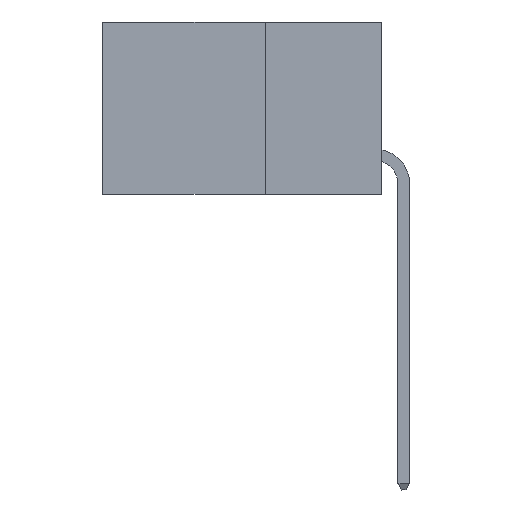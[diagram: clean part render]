
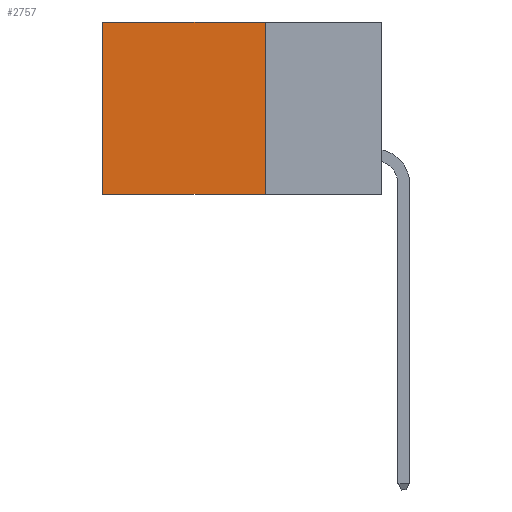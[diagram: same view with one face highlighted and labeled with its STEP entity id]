
A CAD part, left-side view. The second image highlights one B-rep face of the part: STEP entity #2757.
In plain terms, the highlighted planar face has unit normal (-1, 0, 0).
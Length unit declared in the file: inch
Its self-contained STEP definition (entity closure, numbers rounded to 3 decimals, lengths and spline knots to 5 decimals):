
#496 = VECTOR ( 'NONE', #20846, 39.37008 ) ;
#2757 = ADVANCED_FACE ( 'NONE', ( #13807 ), #6725, .F. ) ;
#4314 = DIRECTION ( 'NONE',  ( 0., 1., 0. ) ) ;
#4666 = DIRECTION ( 'NONE',  ( 1., 0., 0. ) ) ;
#4694 = CARTESIAN_POINT ( 'NONE',  ( 0.2875, 0.6, -0.37 ) ) ;
#5157 = CARTESIAN_POINT ( 'NONE',  ( 0.2875, 0.25, -0.37 ) ) ;
#5217 = CARTESIAN_POINT ( 'NONE',  ( 0.2875, 0.6, 0. ) ) ;
#5674 = CARTESIAN_POINT ( 'NONE',  ( 0.2875, 0.25, 0. ) ) ;
#5917 = CARTESIAN_POINT ( 'NONE',  ( 0.2875, 0.25, 0. ) ) ;
#5954 = LINE ( 'NONE', #18958, #496 ) ;
#6725 = PLANE ( 'NONE',  #16886 ) ;
#6920 = LINE ( 'NONE', #5157, #16389 ) ;
#7125 = DIRECTION ( 'NONE',  ( 0., 1., 0. ) ) ;
#7390 = ORIENTED_EDGE ( 'NONE', *, *, #8029, .T. ) ;
#8029 = EDGE_CURVE ( 'NONE', #12331, #22048, #12117, .T. ) ;
#8047 = ORIENTED_EDGE ( 'NONE', *, *, #9166, .T. ) ;
#8820 = DIRECTION ( 'NONE',  ( 0., 0., -1. ) ) ;
#9166 = EDGE_CURVE ( 'NONE', #22048, #13094, #17366, .T. ) ;
#9544 = CARTESIAN_POINT ( 'NONE',  ( 0.2875, 0.6, 0. ) ) ;
#10105 = EDGE_LOOP ( 'NONE', ( #8047, #24276, #16739, #7390 ) ) ;
#11442 = DIRECTION ( 'NONE',  ( 0., 0., -1. ) ) ;
#11542 = VECTOR ( 'NONE', #4314, 39.37008 ) ;
#12117 = LINE ( 'NONE', #17631, #11542 ) ;
#12331 = VERTEX_POINT ( 'NONE', #5917 ) ;
#13094 = VERTEX_POINT ( 'NONE', #4694 ) ;
#13807 = FACE_OUTER_BOUND ( 'NONE', #10105, .T. ) ;
#14584 = EDGE_CURVE ( 'NONE', #19095, #13094, #6920, .T. ) ;
#15245 = EDGE_CURVE ( 'NONE', #12331, #19095, #5954, .T. ) ;
#16175 = VECTOR ( 'NONE', #11442, 39.37008 ) ;
#16389 = VECTOR ( 'NONE', #7125, 39.37008 ) ;
#16739 = ORIENTED_EDGE ( 'NONE', *, *, #15245, .F. ) ;
#16886 = AXIS2_PLACEMENT_3D ( 'NONE', #5674, #4666, #8820 ) ;
#17366 = LINE ( 'NONE', #9544, #16175 ) ;
#17631 = CARTESIAN_POINT ( 'NONE',  ( 0.2875, 0.25, 0. ) ) ;
#18958 = CARTESIAN_POINT ( 'NONE',  ( 0.2875, 0.25, 0. ) ) ;
#19095 = VERTEX_POINT ( 'NONE', #22007 ) ;
#20846 = DIRECTION ( 'NONE',  ( 0., 0., -1. ) ) ;
#22007 = CARTESIAN_POINT ( 'NONE',  ( 0.2875, 0.25, -0.37 ) ) ;
#22048 = VERTEX_POINT ( 'NONE', #5217 ) ;
#24276 = ORIENTED_EDGE ( 'NONE', *, *, #14584, .F. ) ;
